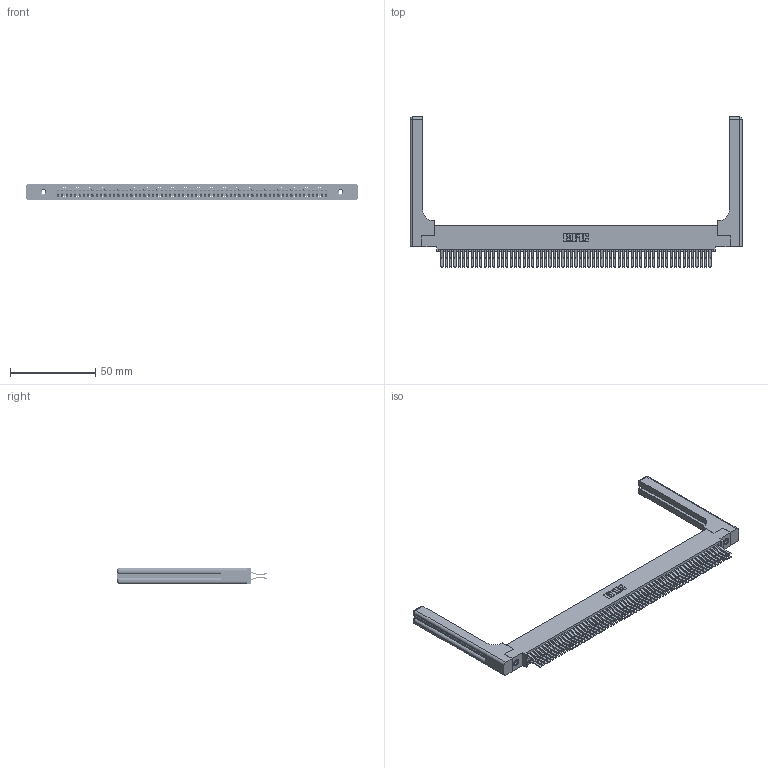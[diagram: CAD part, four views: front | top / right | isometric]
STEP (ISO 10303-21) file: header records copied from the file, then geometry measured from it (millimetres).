
FILE_DESCRIPTION (( 'STEP AP203' ), '1' );
FILE_NAME ('345-126-560-558.STEP', '2019-11-07T06:16:43', ( '' ), ( '' ), 'SwSTEP 2.0', 'SolidWorks 2016', '' );
FILE_SCHEMA (( 'CONFIG_CONTROL_DESIGN' ));
Length unit declared in the file: inch
Products named in the file (5): 345-220-058_345-220-058; 345-126-560-558; 345-292-001_560 Tail; 345-250-001_345-250-001-102; 345 Part_0.110 Offset - 0.156 Dia-TH
Assembly tree (131 placements, depth 2):
  345-126-560-558
    345 Part_0.110 Offset - 0.156 Dia-TH
    345-292-001_560 Tail  x126
    345-250-001_345-250-001-102  x2
    345-220-058_345-220-058  x2
Bounding box: 195.05 x 88.2 x 9.4 mm (x, y, z)
Volume: 28369.6 mm3; surface area: 37089.9 mm2
Topology: 131 solids, 131 shells, 6938 faces, 20549 edges, 13510 vertices
Faces by surface type: plane 4390, cylinder 2488, bspline 36, cone 12, sphere 8, torus 4
Entity records: 52006 total; most frequent: CARTESIAN_POINT 9693, ORIENTED_EDGE 8424, DIRECTION 7456, EDGE_CURVE 4212, LINE 3732, VECTOR 3732, VERTEX_POINT 2798, AXIS2_PLACEMENT_3D 1862
